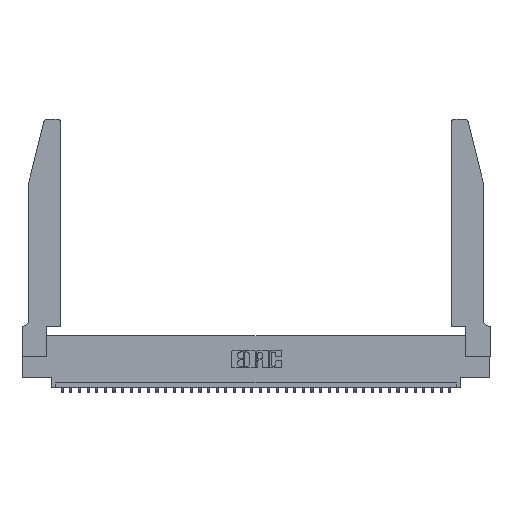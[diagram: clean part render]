
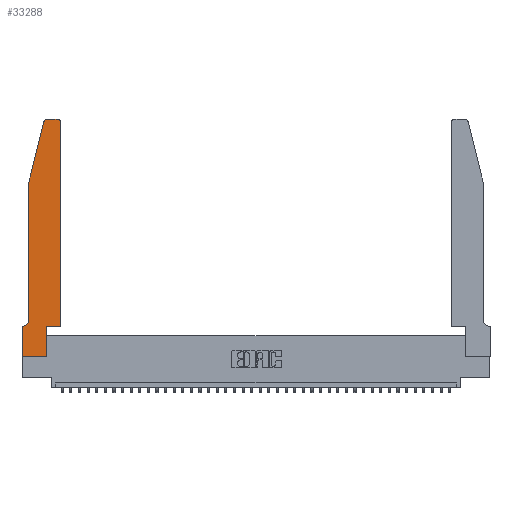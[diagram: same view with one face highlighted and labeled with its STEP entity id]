
A CAD part, top view. The second image highlights one B-rep face of the part: STEP entity #33288.
In plain terms, the highlighted planar face has unit normal (0, 0, 1).
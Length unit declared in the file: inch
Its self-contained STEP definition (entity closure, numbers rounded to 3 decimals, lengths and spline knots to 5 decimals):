
#510 = AXIS2_PLACEMENT_3D ( 'NONE', #10398, #10537, #37695 ) ;
#1079 = VERTEX_POINT ( 'NONE', #4579 ) ;
#1712 = CARTESIAN_POINT ( 'NONE',  ( 0.0755, 2., 0.37 ) ) ;
#2235 = ORIENTED_EDGE ( 'NONE', *, *, #24638, .T. ) ;
#2265 = DIRECTION ( 'NONE',  ( -1., 0., 0. ) ) ;
#2652 = CARTESIAN_POINT ( 'NONE',  ( 0., 0., 0.37 ) ) ;
#3469 = LINE ( 'NONE', #15355, #24683 ) ;
#3802 = VERTEX_POINT ( 'NONE', #38137 ) ;
#3932 = EDGE_CURVE ( 'NONE', #37306, #14813, #25493, .T. ) ;
#4122 = ORIENTED_EDGE ( 'NONE', *, *, #16155, .T. ) ;
#4387 = VERTEX_POINT ( 'NONE', #38477 ) ;
#4579 = CARTESIAN_POINT ( 'NONE',  ( 0.25487, 2.72718, 0.37 ) ) ;
#4667 = VECTOR ( 'NONE', #14464, 39.37008 ) ;
#5022 = DIRECTION ( 'NONE',  ( 0., 0., 1. ) ) ;
#5096 = LINE ( 'NONE', #11288, #36244 ) ;
#5253 = VECTOR ( 'NONE', #2265, 39.37008 ) ;
#5539 = DIRECTION ( 'NONE',  ( 0., 1., 0. ) ) ;
#5802 = ORIENTED_EDGE ( 'NONE', *, *, #39039, .T. ) ;
#6256 = DIRECTION ( 'NONE',  ( 1., 0., 0. ) ) ;
#6298 = CARTESIAN_POINT ( 'NONE',  ( 0.0755, 0.42, 0.37 ) ) ;
#6614 = AXIS2_PLACEMENT_3D ( 'NONE', #38278, #35406, #26684 ) ;
#7108 = LINE ( 'NONE', #24613, #9035 ) ;
#8397 = CARTESIAN_POINT ( 'NONE',  ( 0.4505, 0.35, 0.37 ) ) ;
#9035 = VECTOR ( 'NONE', #27786, 39.37008 ) ;
#9350 = CIRCLE ( 'NONE', #6614, 0.03 ) ;
#9412 = EDGE_CURVE ( 'NONE', #33726, #22457, #7108, .T. ) ;
#9664 = CARTESIAN_POINT ( 'NONE',  ( 0.4505, 2.72, 0.37 ) ) ;
#10243 = ORIENTED_EDGE ( 'NONE', *, *, #11280, .T. ) ;
#10398 = CARTESIAN_POINT ( 'NONE',  ( 0.284, 2.72, 0.37 ) ) ;
#10537 = DIRECTION ( 'NONE',  ( 0., 0., 1. ) ) ;
#10825 = PLANE ( 'NONE',  #18860 ) ;
#10956 = ORIENTED_EDGE ( 'NONE', *, *, #9412, .T. ) ;
#11259 = CARTESIAN_POINT ( 'NONE',  ( 0.0055, 0.42, 0.37 ) ) ;
#11280 = EDGE_CURVE ( 'NONE', #30713, #33726, #20761, .T. ) ;
#11288 = CARTESIAN_POINT ( 'NONE',  ( 0.0755, 0.35, 0.37 ) ) ;
#12703 = ORIENTED_EDGE ( 'NONE', *, *, #3932, .T. ) ;
#12901 = VECTOR ( 'NONE', #20456, 39.37008 ) ;
#13240 = EDGE_LOOP ( 'NONE', ( #27401, #34607, #4122, #17194, #5802, #34850, #12703, #17865, #2235, #10243, #10956, #36069 ) ) ;
#13785 = CARTESIAN_POINT ( 'NONE',  ( 0., 0.35, 0.37 ) ) ;
#13788 = VECTOR ( 'NONE', #34756, 39.37008 ) ;
#13846 = DIRECTION ( 'NONE',  ( 1., 0., 0. ) ) ;
#14003 = EDGE_CURVE ( 'NONE', #4387, #20753, #35187, .T. ) ;
#14464 = DIRECTION ( 'NONE',  ( 1., 0., 0. ) ) ;
#14813 = VERTEX_POINT ( 'NONE', #31415 ) ;
#15355 = CARTESIAN_POINT ( 'NONE',  ( 0., 0., 0.37 ) ) ;
#15431 = CARTESIAN_POINT ( 'NONE',  ( 0.4205, 2.75, 0.37 ) ) ;
#15973 = VECTOR ( 'NONE', #5539, 39.37008 ) ;
#16155 = EDGE_CURVE ( 'NONE', #1079, #4387, #34086, .T. ) ;
#16790 = DIRECTION ( 'NONE',  ( 0., 0., -1. ) ) ;
#16832 = EDGE_CURVE ( 'NONE', #21692, #35876, #29772, .T. ) ;
#16973 = AXIS2_PLACEMENT_3D ( 'NONE', #11259, #16790, #28769 ) ;
#17194 = ORIENTED_EDGE ( 'NONE', *, *, #14003, .T. ) ;
#17865 = ORIENTED_EDGE ( 'NONE', *, *, #22352, .T. ) ;
#17942 = DIRECTION ( 'NONE',  ( 0., -1., 0. ) ) ;
#18860 = AXIS2_PLACEMENT_3D ( 'NONE', #29151, #5022, #13846 ) ;
#18993 = CARTESIAN_POINT ( 'NONE',  ( 0.2865, 0.35, 0.37 ) ) ;
#19209 = CARTESIAN_POINT ( 'NONE',  ( 0.4505, 0.35, 0.37 ) ) ;
#20456 = DIRECTION ( 'NONE',  ( 0., -1., 0. ) ) ;
#20753 = VERTEX_POINT ( 'NONE', #6298 ) ;
#20761 = LINE ( 'NONE', #8397, #4667 ) ;
#21692 = VERTEX_POINT ( 'NONE', #15431 ) ;
#22352 = EDGE_CURVE ( 'NONE', #14813, #25569, #3469, .T. ) ;
#22405 = CIRCLE ( 'NONE', #16973, 0.07 ) ;
#22457 = VERTEX_POINT ( 'NONE', #9664 ) ;
#23606 = LINE ( 'NONE', #18993, #15973 ) ;
#24464 = CARTESIAN_POINT ( 'NONE',  ( 0.2865, 0.35, 0.37 ) ) ;
#24613 = CARTESIAN_POINT ( 'NONE',  ( 0.4505, 0.35, 0.37 ) ) ;
#24638 = EDGE_CURVE ( 'NONE', #25569, #30713, #23606, .T. ) ;
#24683 = VECTOR ( 'NONE', #6256, 39.37008 ) ;
#25276 = EDGE_CURVE ( 'NONE', #22457, #21692, #9350, .T. ) ;
#25493 = LINE ( 'NONE', #2652, #33980 ) ;
#25569 = VERTEX_POINT ( 'NONE', #34695 ) ;
#26684 = DIRECTION ( 'NONE',  ( 1., 0., 0. ) ) ;
#27401 = ORIENTED_EDGE ( 'NONE', *, *, #16832, .T. ) ;
#27786 = DIRECTION ( 'NONE',  ( 0., 1., 0. ) ) ;
#28110 = EDGE_CURVE ( 'NONE', #35876, #1079, #36114, .T. ) ;
#28769 = DIRECTION ( 'NONE',  ( -1., 0., 0. ) ) ;
#29151 = CARTESIAN_POINT ( 'NONE',  ( 0., 0.35, 0.37 ) ) ;
#29409 = CARTESIAN_POINT ( 'NONE',  ( 0.0755, 2., 0.37 ) ) ;
#29772 = LINE ( 'NONE', #38399, #5253 ) ;
#30713 = VERTEX_POINT ( 'NONE', #24464 ) ;
#30732 = FACE_OUTER_BOUND ( 'NONE', #13240, .T. ) ;
#31415 = CARTESIAN_POINT ( 'NONE',  ( 0., 0., 0.37 ) ) ;
#33288 = ADVANCED_FACE ( 'NONE', ( #30732 ), #10825, .T. ) ;
#33726 = VERTEX_POINT ( 'NONE', #19209 ) ;
#33980 = VECTOR ( 'NONE', #17942, 39.37008 ) ;
#34086 = LINE ( 'NONE', #1712, #13788 ) ;
#34607 = ORIENTED_EDGE ( 'NONE', *, *, #28110, .T. ) ;
#34695 = CARTESIAN_POINT ( 'NONE',  ( 0.2865, 0., 0.37 ) ) ;
#34756 = DIRECTION ( 'NONE',  ( -0.239, -0.971, 0. ) ) ;
#34850 = ORIENTED_EDGE ( 'NONE', *, *, #37393, .T. ) ;
#35187 = LINE ( 'NONE', #29409, #12901 ) ;
#35195 = DIRECTION ( 'NONE',  ( -1., 0., 0. ) ) ;
#35406 = DIRECTION ( 'NONE',  ( 0., 0., 1. ) ) ;
#35876 = VERTEX_POINT ( 'NONE', #36548 ) ;
#36069 = ORIENTED_EDGE ( 'NONE', *, *, #25276, .T. ) ;
#36114 = CIRCLE ( 'NONE', #510, 0.03 ) ;
#36244 = VECTOR ( 'NONE', #35195, 39.37008 ) ;
#36548 = CARTESIAN_POINT ( 'NONE',  ( 0.284, 2.75, 0.37 ) ) ;
#37306 = VERTEX_POINT ( 'NONE', #13785 ) ;
#37393 = EDGE_CURVE ( 'NONE', #3802, #37306, #5096, .T. ) ;
#37695 = DIRECTION ( 'NONE',  ( 1., 0., 0. ) ) ;
#38137 = CARTESIAN_POINT ( 'NONE',  ( 0.0055, 0.35, 0.37 ) ) ;
#38278 = CARTESIAN_POINT ( 'NONE',  ( 0.4205, 2.72, 0.37 ) ) ;
#38399 = CARTESIAN_POINT ( 'NONE',  ( 0.2605, 2.75, 0.37 ) ) ;
#38477 = CARTESIAN_POINT ( 'NONE',  ( 0.0755, 2., 0.37 ) ) ;
#39039 = EDGE_CURVE ( 'NONE', #20753, #3802, #22405, .T. ) ;
